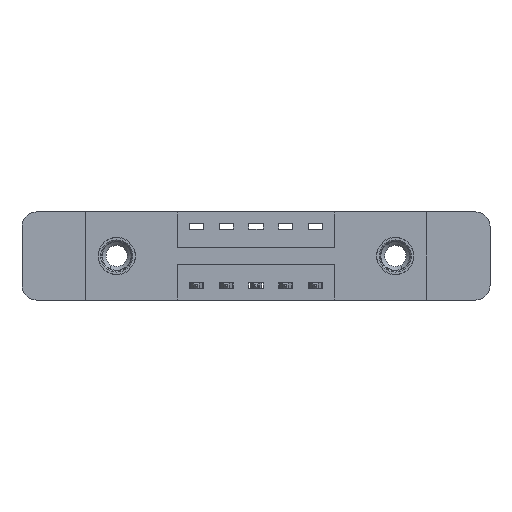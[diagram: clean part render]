
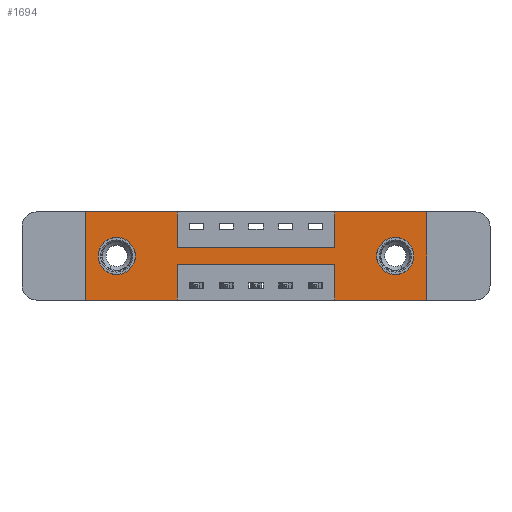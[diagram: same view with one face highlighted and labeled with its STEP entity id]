
A CAD part, front view. The second image highlights one B-rep face of the part: STEP entity #1694.
In plain terms, the highlighted planar face has unit normal (0, -1, 0).
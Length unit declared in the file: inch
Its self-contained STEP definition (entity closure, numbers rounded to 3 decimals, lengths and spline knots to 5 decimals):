
#59 = VECTOR ( 'NONE', #2872, 39.37008 ) ;
#323 = EDGE_CURVE ( 'NONE', #398, #11194, #877, .T. ) ;
#333 = CARTESIAN_POINT ( 'NONE',  ( 0.3875, 0., -0.22 ) ) ;
#398 = VERTEX_POINT ( 'NONE', #12639 ) ;
#435 = EDGE_CURVE ( 'NONE', #2663, #9002, #4607, .T. ) ;
#732 = AXIS2_PLACEMENT_3D ( 'NONE', #13041, #2486, #5703 ) ;
#877 = LINE ( 'NONE', #5136, #6682 ) ;
#878 = EDGE_CURVE ( 'NONE', #12043, #12859, #3782, .T. ) ;
#900 = LINE ( 'NONE', #5159, #2791 ) ;
#939 = CARTESIAN_POINT ( 'NONE',  ( 0., 0., -0.37 ) ) ;
#975 = DIRECTION ( 'NONE',  ( 0., 0., 1. ) ) ;
#982 = ORIENTED_EDGE ( 'NONE', *, *, #11492, .F. ) ;
#1060 = ORIENTED_EDGE ( 'NONE', *, *, #6483, .T. ) ;
#1102 = CIRCLE ( 'NONE', #9962, 0.078 ) ;
#1350 = VECTOR ( 'NONE', #5741, 39.37008 ) ;
#1400 = CIRCLE ( 'NONE', #6062, 0.078 ) ;
#1406 = ORIENTED_EDGE ( 'NONE', *, *, #8405, .T. ) ;
#1440 = LINE ( 'NONE', #9892, #13170 ) ;
#1605 = LINE ( 'NONE', #8967, #59 ) ;
#1694 = ADVANCED_FACE ( 'NONE', ( #4707, #8679, #3660 ), #12912, .T. ) ;
#1782 = LINE ( 'NONE', #10254, #3683 ) ;
#2014 = ORIENTED_EDGE ( 'NONE', *, *, #9257, .F. ) ;
#2017 = CARTESIAN_POINT ( 'NONE',  ( 1.3025, 0., -0.185 ) ) ;
#2486 = DIRECTION ( 'NONE',  ( 0., 1., 0. ) ) ;
#2663 = VERTEX_POINT ( 'NONE', #3031 ) ;
#2791 = VECTOR ( 'NONE', #7305, 39.37008 ) ;
#2872 = DIRECTION ( 'NONE',  ( 1., 0., 0. ) ) ;
#2888 = CARTESIAN_POINT ( 'NONE',  ( 1.0475, 0., -0.22 ) ) ;
#2934 = ORIENTED_EDGE ( 'NONE', *, *, #323, .F. ) ;
#3031 = CARTESIAN_POINT ( 'NONE',  ( 1.0475, 0., -0.37 ) ) ;
#3388 = CIRCLE ( 'NONE', #5843, 0.078 ) ;
#3406 = CARTESIAN_POINT ( 'NONE',  ( 0.3875, 0., -0.37 ) ) ;
#3571 = CARTESIAN_POINT ( 'NONE',  ( 1.0475, 0., -0.37 ) ) ;
#3660 = FACE_OUTER_BOUND ( 'NONE', #3664, .T. ) ;
#3664 = EDGE_LOOP ( 'NONE', ( #13125, #12288, #5889, #13283, #982, #9869, #7488, #6457, #2014, #6604, #2934, #7436 ) ) ;
#3683 = VECTOR ( 'NONE', #4996, 39.37008 ) ;
#3727 = CARTESIAN_POINT ( 'NONE',  ( 1.0475, 0., 0. ) ) ;
#3782 = LINE ( 'NONE', #7900, #4653 ) ;
#4129 = EDGE_CURVE ( 'NONE', #9002, #12043, #9787, .T. ) ;
#4172 = VERTEX_POINT ( 'NONE', #13312 ) ;
#4189 = VERTEX_POINT ( 'NONE', #3727 ) ;
#4458 = EDGE_CURVE ( 'NONE', #11194, #13018, #10931, .T. ) ;
#4489 = VERTEX_POINT ( 'NONE', #10855 ) ;
#4607 = LINE ( 'NONE', #3571, #1350 ) ;
#4630 = LINE ( 'NONE', #13291, #12518 ) ;
#4653 = VECTOR ( 'NONE', #12180, 39.37008 ) ;
#4679 = CARTESIAN_POINT ( 'NONE',  ( 1.3025, 0., -0.263 ) ) ;
#4690 = CARTESIAN_POINT ( 'NONE',  ( 1.3025, 0., -0.185 ) ) ;
#4707 = FACE_BOUND ( 'NONE', #8755, .T. ) ;
#4996 = DIRECTION ( 'NONE',  ( 0., 0., 1. ) ) ;
#5136 = CARTESIAN_POINT ( 'NONE',  ( 0., 0., 0. ) ) ;
#5159 = CARTESIAN_POINT ( 'NONE',  ( 0., 0., -0.37 ) ) ;
#5255 = EDGE_CURVE ( 'NONE', #11752, #2663, #6245, .T. ) ;
#5497 = DIRECTION ( 'NONE',  ( 1., 0., 0. ) ) ;
#5649 = DIRECTION ( 'NONE',  ( -1., 0., 0. ) ) ;
#5697 = CARTESIAN_POINT ( 'NONE',  ( 0.1325, 0., -0.107 ) ) ;
#5703 = DIRECTION ( 'NONE',  ( 0., 0., 1. ) ) ;
#5741 = DIRECTION ( 'NONE',  ( 0., 0., 1. ) ) ;
#5843 = AXIS2_PLACEMENT_3D ( 'NONE', #2017, #8632, #7513 ) ;
#5889 = ORIENTED_EDGE ( 'NONE', *, *, #435, .F. ) ;
#5902 = DIRECTION ( 'NONE',  ( 0., 0., -1. ) ) ;
#5966 = DIRECTION ( 'NONE',  ( 0., 1., 0. ) ) ;
#6062 = AXIS2_PLACEMENT_3D ( 'NONE', #11758, #9587, #975 ) ;
#6245 = LINE ( 'NONE', #939, #9857 ) ;
#6367 = CARTESIAN_POINT ( 'NONE',  ( 0.3875, 0., 0. ) ) ;
#6457 = ORIENTED_EDGE ( 'NONE', *, *, #9084, .F. ) ;
#6483 = EDGE_CURVE ( 'NONE', #4172, #8948, #1102, .T. ) ;
#6510 = ORIENTED_EDGE ( 'NONE', *, *, #8678, .T. ) ;
#6583 = DIRECTION ( 'NONE',  ( 0., 0., -1. ) ) ;
#6604 = ORIENTED_EDGE ( 'NONE', *, *, #4458, .F. ) ;
#6606 = CARTESIAN_POINT ( 'NONE',  ( 0., 0., 0. ) ) ;
#6682 = VECTOR ( 'NONE', #12579, 39.37008 ) ;
#6876 = VERTEX_POINT ( 'NONE', #9120 ) ;
#7111 = CARTESIAN_POINT ( 'NONE',  ( 0., 0., 0. ) ) ;
#7305 = DIRECTION ( 'NONE',  ( -1., 0., 0. ) ) ;
#7415 = EDGE_CURVE ( 'NONE', #4189, #4489, #1605, .T. ) ;
#7436 = ORIENTED_EDGE ( 'NONE', *, *, #11174, .F. ) ;
#7455 = CARTESIAN_POINT ( 'NONE',  ( 0.3875, 0., -0.15 ) ) ;
#7471 = CARTESIAN_POINT ( 'NONE',  ( 0.1325, 0., -0.263 ) ) ;
#7480 = CARTESIAN_POINT ( 'NONE',  ( 1.435, 0., -0.37 ) ) ;
#7488 = ORIENTED_EDGE ( 'NONE', *, *, #12640, .F. ) ;
#7513 = DIRECTION ( 'NONE',  ( 0., 0., -1. ) ) ;
#7702 = DIRECTION ( 'NONE',  ( 0., 0., -1. ) ) ;
#7824 = VECTOR ( 'NONE', #10659, 39.37008 ) ;
#7900 = CARTESIAN_POINT ( 'NONE',  ( 0.3875, 0., -0.37 ) ) ;
#7905 = CARTESIAN_POINT ( 'NONE',  ( 0., 0., -0.37 ) ) ;
#8349 = VECTOR ( 'NONE', #5497, 39.37008 ) ;
#8387 = EDGE_CURVE ( 'NONE', #8948, #4172, #3388, .T. ) ;
#8405 = EDGE_CURVE ( 'NONE', #12614, #10343, #1400, .T. ) ;
#8632 = DIRECTION ( 'NONE',  ( 0., 1., 0. ) ) ;
#8678 = EDGE_CURVE ( 'NONE', #10343, #12614, #9810, .T. ) ;
#8679 = FACE_BOUND ( 'NONE', #13729, .T. ) ;
#8755 = EDGE_LOOP ( 'NONE', ( #1060, #13631 ) ) ;
#8948 = VERTEX_POINT ( 'NONE', #4679 ) ;
#8967 = CARTESIAN_POINT ( 'NONE',  ( 0., 0., 0. ) ) ;
#9002 = VERTEX_POINT ( 'NONE', #2888 ) ;
#9084 = EDGE_CURVE ( 'NONE', #10261, #6876, #12749, .T. ) ;
#9120 = CARTESIAN_POINT ( 'NONE',  ( 1.0475, 0., -0.15 ) ) ;
#9257 = EDGE_CURVE ( 'NONE', #13018, #10261, #4630, .T. ) ;
#9587 = DIRECTION ( 'NONE',  ( 0., 1., 0. ) ) ;
#9780 = DIRECTION ( 'NONE',  ( 0., -1., 0. ) ) ;
#9787 = LINE ( 'NONE', #333, #12549 ) ;
#9810 = CIRCLE ( 'NONE', #732, 0.078 ) ;
#9857 = VECTOR ( 'NONE', #12636, 39.37008 ) ;
#9869 = ORIENTED_EDGE ( 'NONE', *, *, #7415, .F. ) ;
#9892 = CARTESIAN_POINT ( 'NONE',  ( 1.435, 0., 0. ) ) ;
#9962 = AXIS2_PLACEMENT_3D ( 'NONE', #4690, #5966, #10100 ) ;
#10100 = DIRECTION ( 'NONE',  ( 0., 0., -1. ) ) ;
#10247 = CARTESIAN_POINT ( 'NONE',  ( 0.3875, 0., -0.15 ) ) ;
#10254 = CARTESIAN_POINT ( 'NONE',  ( 1.0475, 0., 0. ) ) ;
#10261 = VERTEX_POINT ( 'NONE', #10247 ) ;
#10343 = VERTEX_POINT ( 'NONE', #7471 ) ;
#10659 = DIRECTION ( 'NONE',  ( 1., 0., 0. ) ) ;
#10855 = CARTESIAN_POINT ( 'NONE',  ( 1.435, 0., 0. ) ) ;
#10924 = AXIS2_PLACEMENT_3D ( 'NONE', #7905, #9780, #7702 ) ;
#10931 = LINE ( 'NONE', #6606, #8349 ) ;
#11174 = EDGE_CURVE ( 'NONE', #12859, #398, #900, .T. ) ;
#11194 = VERTEX_POINT ( 'NONE', #7111 ) ;
#11492 = EDGE_CURVE ( 'NONE', #4489, #11752, #1440, .T. ) ;
#11752 = VERTEX_POINT ( 'NONE', #7480 ) ;
#11758 = CARTESIAN_POINT ( 'NONE',  ( 0.1325, 0., -0.185 ) ) ;
#12043 = VERTEX_POINT ( 'NONE', #13577 ) ;
#12180 = DIRECTION ( 'NONE',  ( 0., 0., -1. ) ) ;
#12288 = ORIENTED_EDGE ( 'NONE', *, *, #4129, .F. ) ;
#12518 = VECTOR ( 'NONE', #5902, 39.37008 ) ;
#12549 = VECTOR ( 'NONE', #5649, 39.37008 ) ;
#12579 = DIRECTION ( 'NONE',  ( 0., 0., 1. ) ) ;
#12614 = VERTEX_POINT ( 'NONE', #5697 ) ;
#12636 = DIRECTION ( 'NONE',  ( -1., 0., 0. ) ) ;
#12639 = CARTESIAN_POINT ( 'NONE',  ( 0., 0., -0.37 ) ) ;
#12640 = EDGE_CURVE ( 'NONE', #6876, #4189, #1782, .T. ) ;
#12749 = LINE ( 'NONE', #7455, #7824 ) ;
#12859 = VERTEX_POINT ( 'NONE', #3406 ) ;
#12912 = PLANE ( 'NONE',  #10924 ) ;
#13018 = VERTEX_POINT ( 'NONE', #6367 ) ;
#13041 = CARTESIAN_POINT ( 'NONE',  ( 0.1325, 0., -0.185 ) ) ;
#13125 = ORIENTED_EDGE ( 'NONE', *, *, #878, .F. ) ;
#13170 = VECTOR ( 'NONE', #6583, 39.37008 ) ;
#13283 = ORIENTED_EDGE ( 'NONE', *, *, #5255, .F. ) ;
#13291 = CARTESIAN_POINT ( 'NONE',  ( 0.3875, 0., 0. ) ) ;
#13312 = CARTESIAN_POINT ( 'NONE',  ( 1.3025, 0., -0.107 ) ) ;
#13577 = CARTESIAN_POINT ( 'NONE',  ( 0.3875, 0., -0.22 ) ) ;
#13631 = ORIENTED_EDGE ( 'NONE', *, *, #8387, .T. ) ;
#13729 = EDGE_LOOP ( 'NONE', ( #1406, #6510 ) ) ;
